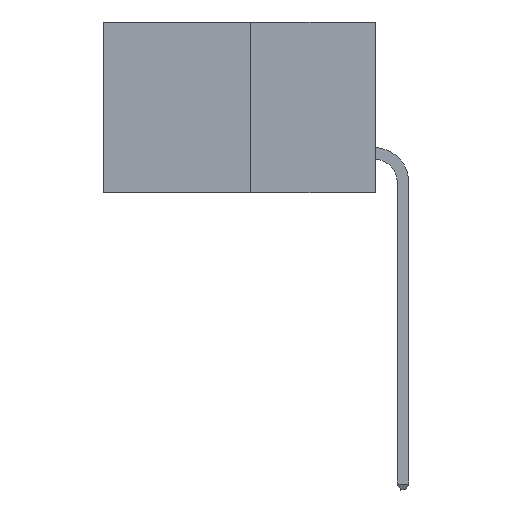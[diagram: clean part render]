
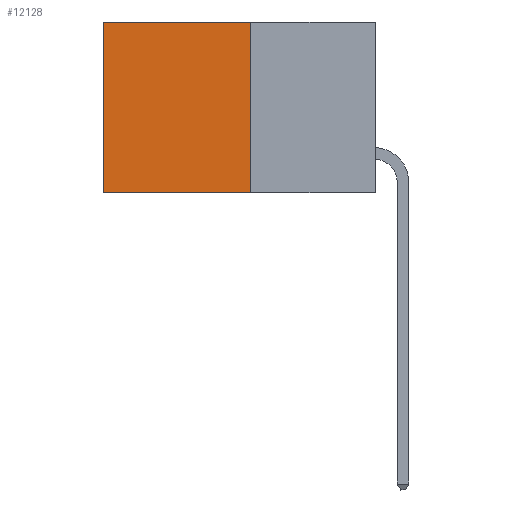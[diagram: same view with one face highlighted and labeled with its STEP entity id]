
A CAD part, left-side view. The second image highlights one B-rep face of the part: STEP entity #12128.
In plain terms, the highlighted planar face has unit normal (-1, 0, 0).
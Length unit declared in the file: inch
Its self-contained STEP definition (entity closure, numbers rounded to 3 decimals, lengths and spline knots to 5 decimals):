
#848 = EDGE_CURVE ( 'NONE', #7275, #8914, #8131, .T. ) ;
#1003 = LINE ( 'NONE', #22253, #10416 ) ;
#1506 = CARTESIAN_POINT ( 'NONE',  ( 0.277, 0.27, -0.37 ) ) ;
#1589 = DIRECTION ( 'NONE',  ( 0., 0., -1. ) ) ;
#2442 = CARTESIAN_POINT ( 'NONE',  ( 0.277, 0.27, 0. ) ) ;
#2638 = CARTESIAN_POINT ( 'NONE',  ( 0.277, 0.59, -0.37 ) ) ;
#2811 = EDGE_CURVE ( 'NONE', #12487, #8914, #1003, .T. ) ;
#3260 = CARTESIAN_POINT ( 'NONE',  ( 0.277, 0.27, 0. ) ) ;
#3339 = CARTESIAN_POINT ( 'NONE',  ( 0.277, 0.59, 0. ) ) ;
#4519 = ORIENTED_EDGE ( 'NONE', *, *, #13732, .T. ) ;
#4828 = ORIENTED_EDGE ( 'NONE', *, *, #848, .T. ) ;
#5085 = CARTESIAN_POINT ( 'NONE',  ( 0.277, 0.27, -0.37 ) ) ;
#6524 = DIRECTION ( 'NONE',  ( 0., 1., 0. ) ) ;
#7275 = VERTEX_POINT ( 'NONE', #3339 ) ;
#7865 = EDGE_LOOP ( 'NONE', ( #4828, #15157, #16688, #4519 ) ) ;
#7900 = VECTOR ( 'NONE', #14033, 39.37008 ) ;
#8131 = LINE ( 'NONE', #18317, #7900 ) ;
#8914 = VERTEX_POINT ( 'NONE', #2638 ) ;
#9316 = VECTOR ( 'NONE', #21355, 39.37008 ) ;
#10416 = VECTOR ( 'NONE', #6524, 39.37008 ) ;
#12057 = DIRECTION ( 'NONE',  ( 1., 0., 0. ) ) ;
#12128 = ADVANCED_FACE ( 'NONE', ( #20982 ), #22222, .F. ) ;
#12487 = VERTEX_POINT ( 'NONE', #13294 ) ;
#12921 = AXIS2_PLACEMENT_3D ( 'NONE', #1506, #12057, #1589 ) ;
#13294 = CARTESIAN_POINT ( 'NONE',  ( 0.277, 0.27, -0.37 ) ) ;
#13732 = EDGE_CURVE ( 'NONE', #18459, #7275, #15463, .T. ) ;
#13783 = LINE ( 'NONE', #5085, #17805 ) ;
#14033 = DIRECTION ( 'NONE',  ( 0., 0., -1. ) ) ;
#14976 = EDGE_CURVE ( 'NONE', #18459, #12487, #13783, .T. ) ;
#15157 = ORIENTED_EDGE ( 'NONE', *, *, #2811, .F. ) ;
#15458 = DIRECTION ( 'NONE',  ( 0., 0., -1. ) ) ;
#15463 = LINE ( 'NONE', #2442, #9316 ) ;
#16688 = ORIENTED_EDGE ( 'NONE', *, *, #14976, .F. ) ;
#17805 = VECTOR ( 'NONE', #15458, 39.37008 ) ;
#18317 = CARTESIAN_POINT ( 'NONE',  ( 0.277, 0.59, -0.37 ) ) ;
#18459 = VERTEX_POINT ( 'NONE', #3260 ) ;
#20982 = FACE_OUTER_BOUND ( 'NONE', #7865, .T. ) ;
#21355 = DIRECTION ( 'NONE',  ( 0., 1., 0. ) ) ;
#22222 = PLANE ( 'NONE',  #12921 ) ;
#22253 = CARTESIAN_POINT ( 'NONE',  ( 0.277, 0.27, -0.37 ) ) ;
